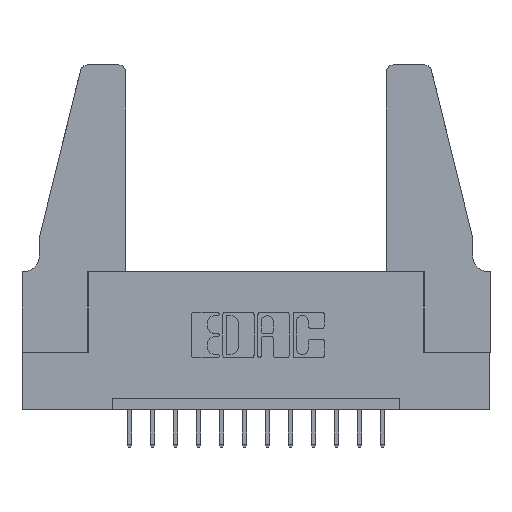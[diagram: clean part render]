
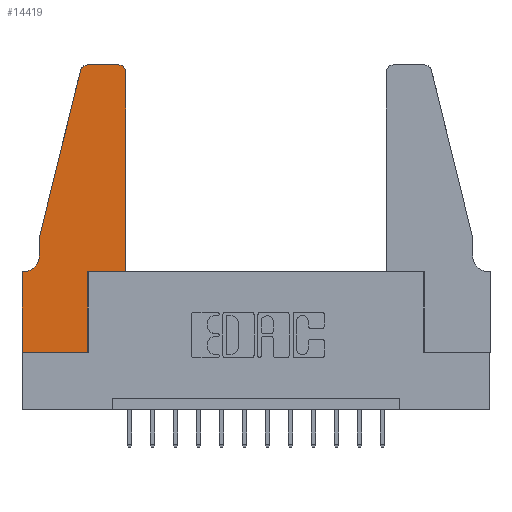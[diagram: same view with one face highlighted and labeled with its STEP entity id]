
A CAD part, top view. The second image highlights one B-rep face of the part: STEP entity #14419.
In plain terms, the highlighted planar face has unit normal (0, 0, 1).
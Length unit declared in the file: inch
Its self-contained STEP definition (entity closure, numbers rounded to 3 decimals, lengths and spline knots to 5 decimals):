
#259 = VECTOR ( 'NONE', #11738, 39.37008 ) ;
#517 = DIRECTION ( 'NONE',  ( 0., -1., 0. ) ) ;
#558 = DIRECTION ( 'NONE',  ( 0., -1., 0. ) ) ;
#595 = VERTEX_POINT ( 'NONE', #11063 ) ;
#674 = CARTESIAN_POINT ( 'NONE',  ( 0.0755, 0.5, 0.37 ) ) ;
#878 = VERTEX_POINT ( 'NONE', #5468 ) ;
#1054 = DIRECTION ( 'NONE',  ( 1., 0., 0. ) ) ;
#1310 = EDGE_CURVE ( 'NONE', #5927, #9342, #10281, .T. ) ;
#1568 = LINE ( 'NONE', #11725, #1959 ) ;
#1611 = CARTESIAN_POINT ( 'NONE',  ( 0., 0., 0.37 ) ) ;
#1685 = LINE ( 'NONE', #11269, #2418 ) ;
#1940 = CARTESIAN_POINT ( 'NONE',  ( 0.4205, 1.25, 0.37 ) ) ;
#1959 = VECTOR ( 'NONE', #8063, 39.37008 ) ;
#2063 = CARTESIAN_POINT ( 'NONE',  ( 0.2865, 0.35, 0.37 ) ) ;
#2190 = CARTESIAN_POINT ( 'NONE',  ( 0., 0.35, 0.37 ) ) ;
#2270 = LINE ( 'NONE', #8020, #3022 ) ;
#2418 = VECTOR ( 'NONE', #517, 39.37008 ) ;
#2461 = CIRCLE ( 'NONE', #6233, 0.03 ) ;
#2600 = VECTOR ( 'NONE', #14659, 39.37008 ) ;
#2825 = CARTESIAN_POINT ( 'NONE',  ( 0., 0.35, 0.37 ) ) ;
#3022 = VECTOR ( 'NONE', #1054, 39.37008 ) ;
#3117 = ORIENTED_EDGE ( 'NONE', *, *, #7258, .T. ) ;
#3285 = VECTOR ( 'NONE', #10897, 39.37008 ) ;
#3559 = DIRECTION ( 'NONE',  ( 0., 0., 1. ) ) ;
#3605 = ORIENTED_EDGE ( 'NONE', *, *, #7519, .T. ) ;
#3707 = ORIENTED_EDGE ( 'NONE', *, *, #13179, .T. ) ;
#3872 = VECTOR ( 'NONE', #5222, 39.37008 ) ;
#4136 = CARTESIAN_POINT ( 'NONE',  ( 0.0755, 0.35, 0.37 ) ) ;
#4253 = LINE ( 'NONE', #4136, #3872 ) ;
#4420 = EDGE_CURVE ( 'NONE', #10352, #6626, #2461, .T. ) ;
#4587 = EDGE_CURVE ( 'NONE', #878, #8028, #2270, .T. ) ;
#4838 = CARTESIAN_POINT ( 'NONE',  ( 0.0755, 0.42, 0.37 ) ) ;
#5131 = CIRCLE ( 'NONE', #8255, 0.03 ) ;
#5222 = DIRECTION ( 'NONE',  ( -1., 0., 0. ) ) ;
#5268 = DIRECTION ( 'NONE',  ( 0., 0., 1. ) ) ;
#5387 = CARTESIAN_POINT ( 'NONE',  ( 0.4505, 0.35, 0.37 ) ) ;
#5468 = CARTESIAN_POINT ( 'NONE',  ( 0.2865, 0.35, 0.37 ) ) ;
#5607 = ORIENTED_EDGE ( 'NONE', *, *, #4587, .T. ) ;
#5678 = DIRECTION ( 'NONE',  ( 1., 0., 0. ) ) ;
#5927 = VERTEX_POINT ( 'NONE', #4838 ) ;
#6051 = CARTESIAN_POINT ( 'NONE',  ( 0.2865, 0., 0.37 ) ) ;
#6111 = ORIENTED_EDGE ( 'NONE', *, *, #6619, .T. ) ;
#6176 = VERTEX_POINT ( 'NONE', #13621 ) ;
#6233 = AXIS2_PLACEMENT_3D ( 'NONE', #13777, #14919, #13673 ) ;
#6302 = EDGE_CURVE ( 'NONE', #13329, #10352, #7697, .T. ) ;
#6404 = LINE ( 'NONE', #674, #12290 ) ;
#6441 = DIRECTION ( 'NONE',  ( 1., 0., 0. ) ) ;
#6619 = EDGE_CURVE ( 'NONE', #6626, #6724, #12475, .T. ) ;
#6626 = VERTEX_POINT ( 'NONE', #9246 ) ;
#6724 = VERTEX_POINT ( 'NONE', #6813 ) ;
#6813 = CARTESIAN_POINT ( 'NONE',  ( 0.0755, 0.5, 0.37 ) ) ;
#6855 = LINE ( 'NONE', #1611, #2600 ) ;
#7000 = FACE_OUTER_BOUND ( 'NONE', #14111, .T. ) ;
#7158 = CARTESIAN_POINT ( 'NONE',  ( 0.0055, 0.42, 0.37 ) ) ;
#7258 = EDGE_CURVE ( 'NONE', #6724, #5927, #6404, .T. ) ;
#7355 = ORIENTED_EDGE ( 'NONE', *, *, #6302, .T. ) ;
#7519 = EDGE_CURVE ( 'NONE', #8028, #6176, #1568, .T. ) ;
#7697 = LINE ( 'NONE', #9636, #3285 ) ;
#7709 = ORIENTED_EDGE ( 'NONE', *, *, #9626, .T. ) ;
#7858 = ORIENTED_EDGE ( 'NONE', *, *, #15298, .T. ) ;
#8020 = CARTESIAN_POINT ( 'NONE',  ( 0.4505, 0.35, 0.37 ) ) ;
#8028 = VERTEX_POINT ( 'NONE', #5387 ) ;
#8063 = DIRECTION ( 'NONE',  ( 0., 1., 0. ) ) ;
#8255 = AXIS2_PLACEMENT_3D ( 'NONE', #9388, #3559, #5678 ) ;
#8281 = CARTESIAN_POINT ( 'NONE',  ( 0.0055, 0.35, 0.37 ) ) ;
#8628 = VECTOR ( 'NONE', #10145, 39.37008 ) ;
#9143 = AXIS2_PLACEMENT_3D ( 'NONE', #7158, #12928, #11750 ) ;
#9239 = CARTESIAN_POINT ( 'NONE',  ( 0.0755, 0.5, 0.37 ) ) ;
#9246 = CARTESIAN_POINT ( 'NONE',  ( 0.25487, 1.22718, 0.37 ) ) ;
#9342 = VERTEX_POINT ( 'NONE', #8281 ) ;
#9388 = CARTESIAN_POINT ( 'NONE',  ( 0.4205, 1.22, 0.37 ) ) ;
#9626 = EDGE_CURVE ( 'NONE', #595, #11142, #6855, .T. ) ;
#9636 = CARTESIAN_POINT ( 'NONE',  ( 0.2605, 1.25, 0.37 ) ) ;
#9730 = LINE ( 'NONE', #2063, #8628 ) ;
#9820 = AXIS2_PLACEMENT_3D ( 'NONE', #2825, #5268, #6441 ) ;
#10145 = DIRECTION ( 'NONE',  ( 0., 1., 0. ) ) ;
#10281 = CIRCLE ( 'NONE', #9143, 0.07 ) ;
#10352 = VERTEX_POINT ( 'NONE', #13342 ) ;
#10897 = DIRECTION ( 'NONE',  ( -1., 0., 0. ) ) ;
#11063 = CARTESIAN_POINT ( 'NONE',  ( 0., 0., 0.37 ) ) ;
#11142 = VERTEX_POINT ( 'NONE', #6051 ) ;
#11177 = PLANE ( 'NONE',  #9820 ) ;
#11265 = ORIENTED_EDGE ( 'NONE', *, *, #14432, .T. ) ;
#11269 = CARTESIAN_POINT ( 'NONE',  ( 0., 0., 0.37 ) ) ;
#11524 = EDGE_CURVE ( 'NONE', #11142, #878, #9730, .T. ) ;
#11725 = CARTESIAN_POINT ( 'NONE',  ( 0.4505, 0.35, 0.37 ) ) ;
#11738 = DIRECTION ( 'NONE',  ( -0.239, -0.971, 0. ) ) ;
#11750 = DIRECTION ( 'NONE',  ( -1., 0., 0. ) ) ;
#12290 = VECTOR ( 'NONE', #558, 39.37008 ) ;
#12314 = VERTEX_POINT ( 'NONE', #2190 ) ;
#12475 = LINE ( 'NONE', #9239, #259 ) ;
#12751 = ORIENTED_EDGE ( 'NONE', *, *, #1310, .T. ) ;
#12928 = DIRECTION ( 'NONE',  ( 0., 0., -1. ) ) ;
#13179 = EDGE_CURVE ( 'NONE', #12314, #595, #1685, .T. ) ;
#13329 = VERTEX_POINT ( 'NONE', #1940 ) ;
#13342 = CARTESIAN_POINT ( 'NONE',  ( 0.284, 1.25, 0.37 ) ) ;
#13468 = ORIENTED_EDGE ( 'NONE', *, *, #4420, .T. ) ;
#13621 = CARTESIAN_POINT ( 'NONE',  ( 0.4505, 1.22, 0.37 ) ) ;
#13673 = DIRECTION ( 'NONE',  ( 1., 0., 0. ) ) ;
#13777 = CARTESIAN_POINT ( 'NONE',  ( 0.284, 1.22, 0.37 ) ) ;
#14111 = EDGE_LOOP ( 'NONE', ( #7355, #13468, #6111, #3117, #12751, #11265, #3707, #7709, #15006, #5607, #3605, #7858 ) ) ;
#14419 = ADVANCED_FACE ( 'NONE', ( #7000 ), #11177, .T. ) ;
#14432 = EDGE_CURVE ( 'NONE', #9342, #12314, #4253, .T. ) ;
#14659 = DIRECTION ( 'NONE',  ( 1., 0., 0. ) ) ;
#14919 = DIRECTION ( 'NONE',  ( 0., 0., 1. ) ) ;
#15006 = ORIENTED_EDGE ( 'NONE', *, *, #11524, .T. ) ;
#15298 = EDGE_CURVE ( 'NONE', #6176, #13329, #5131, .T. ) ;
